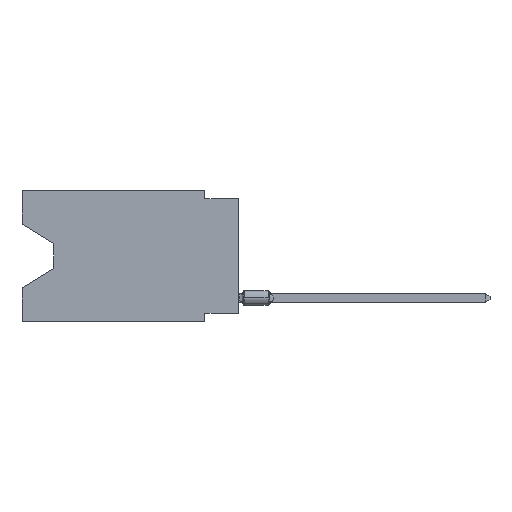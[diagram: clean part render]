
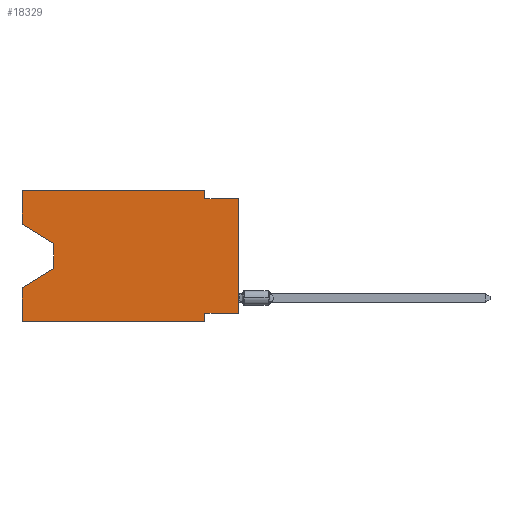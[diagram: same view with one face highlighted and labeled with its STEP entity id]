
A CAD part, left-side view. The second image highlights one B-rep face of the part: STEP entity #18329.
In plain terms, the highlighted planar face has unit normal (-1, 0, 0).
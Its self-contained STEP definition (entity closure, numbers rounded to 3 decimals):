
#255 = ORIENTED_EDGE ( 'NONE', *, *, #17747, .T. ) ;
#666 = EDGE_CURVE ( 'NONE', #21015, #22000, #28909, .T. ) ;
#889 = EDGE_CURVE ( 'NONE', #10140, #5780, #21771, .T. ) ;
#1597 = CARTESIAN_POINT ( 'NONE',  ( 0., 16.383, 0. ) ) ;
#1868 = ORIENTED_EDGE ( 'NONE', *, *, #889, .F. ) ;
#1890 = LINE ( 'NONE', #1597, #21695 ) ;
#2329 = CARTESIAN_POINT ( 'NONE',  ( 0., 13.97, -4.013 ) ) ;
#2774 = CARTESIAN_POINT ( 'NONE',  ( 0., 2.54, 0. ) ) ;
#2808 = EDGE_CURVE ( 'NONE', #10140, #25293, #27049, .T. ) ;
#2921 = CARTESIAN_POINT ( 'NONE',  ( 0., 16.383, -9.906 ) ) ;
#2951 = CARTESIAN_POINT ( 'NONE',  ( 0., 16.383, -9.906 ) ) ;
#3416 = LINE ( 'NONE', #12420, #4880 ) ;
#4294 = DIRECTION ( 'NONE',  ( 0., 0., 1. ) ) ;
#4526 = CARTESIAN_POINT ( 'NONE',  ( 0., 13.97, -5.893 ) ) ;
#4624 = VERTEX_POINT ( 'NONE', #17160 ) ;
#4880 = VECTOR ( 'NONE', #5191, 1000. ) ;
#4991 = ORIENTED_EDGE ( 'NONE', *, *, #17085, .T. ) ;
#5191 = DIRECTION ( 'NONE',  ( 0., 1., 0. ) ) ;
#5597 = ORIENTED_EDGE ( 'NONE', *, *, #11309, .F. ) ;
#5780 = VERTEX_POINT ( 'NONE', #16619 ) ;
#6071 = VECTOR ( 'NONE', #28063, 1000. ) ;
#6082 = DIRECTION ( 'NONE',  ( 0., 0., -1. ) ) ;
#6952 = CARTESIAN_POINT ( 'NONE',  ( 0., 16.383, -2.546 ) ) ;
#8216 = CARTESIAN_POINT ( 'NONE',  ( 0., 16.383, 0. ) ) ;
#8498 = VERTEX_POINT ( 'NONE', #10607 ) ;
#8590 = CARTESIAN_POINT ( 'NONE',  ( 0., 2.54, -9.906 ) ) ;
#8635 = DIRECTION ( 'NONE',  ( 0., -0.855, -0.519 ) ) ;
#10066 = ORIENTED_EDGE ( 'NONE', *, *, #23882, .F. ) ;
#10088 = VERTEX_POINT ( 'NONE', #23305 ) ;
#10140 = VERTEX_POINT ( 'NONE', #2921 ) ;
#10158 = CARTESIAN_POINT ( 'NONE',  ( 0., 2.54, -0.635 ) ) ;
#10199 = VECTOR ( 'NONE', #27488, 1000. ) ;
#10224 = ORIENTED_EDGE ( 'NONE', *, *, #2808, .T. ) ;
#10241 = ORIENTED_EDGE ( 'NONE', *, *, #13404, .T. ) ;
#10607 = CARTESIAN_POINT ( 'NONE',  ( 0., 2.54, 0. ) ) ;
#10642 = LINE ( 'NONE', #19666, #20717 ) ;
#11076 = CARTESIAN_POINT ( 'NONE',  ( 0., 0., 0. ) ) ;
#11309 = EDGE_CURVE ( 'NONE', #25136, #25293, #28551, .T. ) ;
#11345 = DIRECTION ( 'NONE',  ( 0., 0., -1. ) ) ;
#12420 = CARTESIAN_POINT ( 'NONE',  ( 0., 0., -9.271 ) ) ;
#13226 = EDGE_CURVE ( 'NONE', #8498, #21015, #18444, .T. ) ;
#13404 = EDGE_CURVE ( 'NONE', #21680, #10088, #19872, .T. ) ;
#13430 = VECTOR ( 'NONE', #8635, 1000. ) ;
#13567 = CARTESIAN_POINT ( 'NONE',  ( 0., 16.383, 0. ) ) ;
#14075 = EDGE_CURVE ( 'NONE', #17829, #25136, #3416, .T. ) ;
#14295 = VERTEX_POINT ( 'NONE', #13567 ) ;
#14687 = CARTESIAN_POINT ( 'NONE',  ( 0., 16.383, 0. ) ) ;
#15013 = DIRECTION ( 'NONE',  ( 1., 0., 0. ) ) ;
#15573 = CARTESIAN_POINT ( 'NONE',  ( 0., 16.383, -2.546 ) ) ;
#15668 = LINE ( 'NONE', #11076, #22304 ) ;
#16619 = CARTESIAN_POINT ( 'NONE',  ( 0., 16.383, -7.36 ) ) ;
#16620 = DIRECTION ( 'NONE',  ( 0., 0., 1. ) ) ;
#17085 = EDGE_CURVE ( 'NONE', #4624, #5780, #20494, .T. ) ;
#17160 = CARTESIAN_POINT ( 'NONE',  ( 0., 13.97, -5.893 ) ) ;
#17747 = EDGE_CURVE ( 'NONE', #17829, #22000, #15668, .T. ) ;
#17821 = ORIENTED_EDGE ( 'NONE', *, *, #23615, .F. ) ;
#17829 = VERTEX_POINT ( 'NONE', #23197 ) ;
#18311 = VECTOR ( 'NONE', #19726, 1000. ) ;
#18329 = ADVANCED_FACE ( 'NONE', ( #27902 ), #26109, .F. ) ;
#18444 = LINE ( 'NONE', #2774, #6071 ) ;
#18898 = ORIENTED_EDGE ( 'NONE', *, *, #666, .F. ) ;
#18965 = VECTOR ( 'NONE', #24763, 1000. ) ;
#19161 = DIRECTION ( 'NONE',  ( 0., 0., -1. ) ) ;
#19666 = CARTESIAN_POINT ( 'NONE',  ( 0., 16.383, 0. ) ) ;
#19726 = DIRECTION ( 'NONE',  ( 0., -1., 0. ) ) ;
#19872 = LINE ( 'NONE', #15573, #13430 ) ;
#19905 = AXIS2_PLACEMENT_3D ( 'NONE', #8216, #15013, #19161 ) ;
#20494 = LINE ( 'NONE', #4526, #18965 ) ;
#20505 = LINE ( 'NONE', #2329, #21739 ) ;
#20696 = VECTOR ( 'NONE', #16620, 1000. ) ;
#20717 = VECTOR ( 'NONE', #22599, 1000. ) ;
#21015 = VERTEX_POINT ( 'NONE', #10158 ) ;
#21256 = CARTESIAN_POINT ( 'NONE',  ( 0., 2.54, -9.906 ) ) ;
#21680 = VERTEX_POINT ( 'NONE', #6952 ) ;
#21695 = VECTOR ( 'NONE', #21993, 1000. ) ;
#21739 = VECTOR ( 'NONE', #11345, 1000. ) ;
#21771 = LINE ( 'NONE', #14687, #20696 ) ;
#21854 = ORIENTED_EDGE ( 'NONE', *, *, #27143, .T. ) ;
#21993 = DIRECTION ( 'NONE',  ( 0., 0., 1. ) ) ;
#22000 = VERTEX_POINT ( 'NONE', #27038 ) ;
#22148 = ORIENTED_EDGE ( 'NONE', *, *, #13226, .F. ) ;
#22304 = VECTOR ( 'NONE', #4294, 1000. ) ;
#22379 = CARTESIAN_POINT ( 'NONE',  ( 0., 0., -0.635 ) ) ;
#22426 = CARTESIAN_POINT ( 'NONE',  ( 0., 2.54, -9.271 ) ) ;
#22599 = DIRECTION ( 'NONE',  ( 0., -1., 0. ) ) ;
#23197 = CARTESIAN_POINT ( 'NONE',  ( 0., 0., -9.271 ) ) ;
#23305 = CARTESIAN_POINT ( 'NONE',  ( 0., 13.97, -4.013 ) ) ;
#23615 = EDGE_CURVE ( 'NONE', #14295, #8498, #10642, .T. ) ;
#23882 = EDGE_CURVE ( 'NONE', #21680, #14295, #1890, .T. ) ;
#24763 = DIRECTION ( 'NONE',  ( 0., 0.855, -0.519 ) ) ;
#25136 = VERTEX_POINT ( 'NONE', #22426 ) ;
#25293 = VERTEX_POINT ( 'NONE', #21256 ) ;
#25577 = EDGE_LOOP ( 'NONE', ( #10241, #21854, #4991, #1868, #10224, #5597, #26724, #255, #18898, #22148, #17821, #10066 ) ) ;
#26109 = PLANE ( 'NONE',  #19905 ) ;
#26724 = ORIENTED_EDGE ( 'NONE', *, *, #14075, .F. ) ;
#27038 = CARTESIAN_POINT ( 'NONE',  ( 0., 0., -0.635 ) ) ;
#27049 = LINE ( 'NONE', #2951, #10199 ) ;
#27143 = EDGE_CURVE ( 'NONE', #10088, #4624, #20505, .T. ) ;
#27220 = VECTOR ( 'NONE', #6082, 1000. ) ;
#27488 = DIRECTION ( 'NONE',  ( 0., -1., 0. ) ) ;
#27902 = FACE_OUTER_BOUND ( 'NONE', #25577, .T. ) ;
#28063 = DIRECTION ( 'NONE',  ( 0., 0., -1. ) ) ;
#28551 = LINE ( 'NONE', #8590, #27220 ) ;
#28909 = LINE ( 'NONE', #22379, #18311 ) ;
